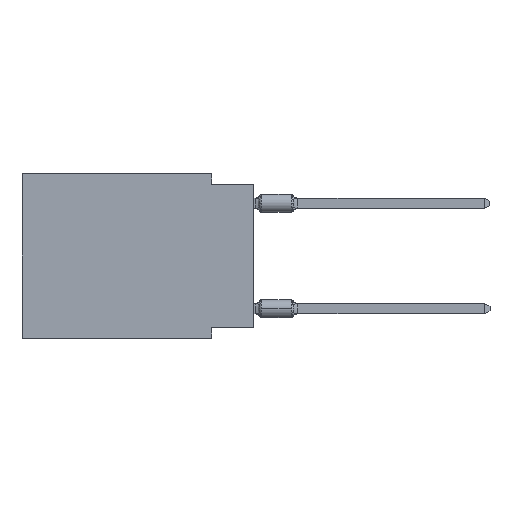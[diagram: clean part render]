
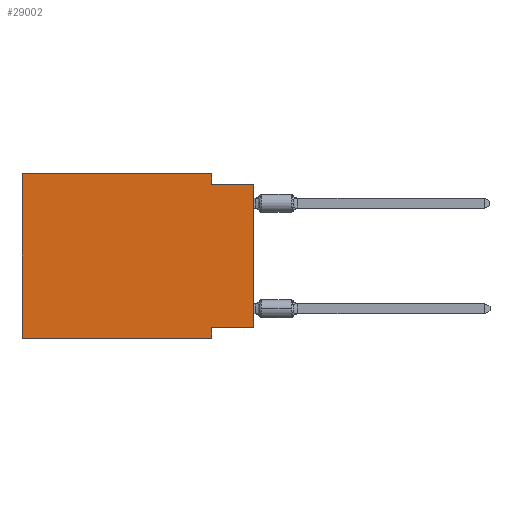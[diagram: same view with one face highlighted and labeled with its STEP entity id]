
A CAD part, left-side view. The second image highlights one B-rep face of the part: STEP entity #29002.
In plain terms, the highlighted planar face has unit normal (-1, 0, 0).
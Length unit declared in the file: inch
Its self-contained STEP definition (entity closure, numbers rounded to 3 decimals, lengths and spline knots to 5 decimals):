
#120 = CARTESIAN_POINT ( 'NONE',  ( 0., 0.1, -0.365 ) ) ;
#843 = DIRECTION ( 'NONE',  ( 0., -1., 0. ) ) ;
#1468 = CARTESIAN_POINT ( 'NONE',  ( 0., 0., -0.365 ) ) ;
#3366 = VERTEX_POINT ( 'NONE', #50216 ) ;
#4044 = LINE ( 'NONE', #29016, #26441 ) ;
#4086 = CARTESIAN_POINT ( 'NONE',  ( 0., 0., 0. ) ) ;
#5196 = CARTESIAN_POINT ( 'NONE',  ( 0., 0.55, 0. ) ) ;
#5361 = LINE ( 'NONE', #50128, #23396 ) ;
#6014 = ORIENTED_EDGE ( 'NONE', *, *, #18620, .T. ) ;
#8143 = CARTESIAN_POINT ( 'NONE',  ( 0., 0.55, 0. ) ) ;
#9577 = LINE ( 'NONE', #39129, #50438 ) ;
#12349 = ORIENTED_EDGE ( 'NONE', *, *, #35644, .F. ) ;
#12462 = VERTEX_POINT ( 'NONE', #38360 ) ;
#12705 = CARTESIAN_POINT ( 'NONE',  ( 0., 0., -0.365 ) ) ;
#13764 = DIRECTION ( 'NONE',  ( 0., 0., 1. ) ) ;
#14837 = PLANE ( 'NONE',  #52982 ) ;
#15242 = VERTEX_POINT ( 'NONE', #12705 ) ;
#15736 = LINE ( 'NONE', #8143, #47557 ) ;
#16012 = CARTESIAN_POINT ( 'NONE',  ( 0., 0.1, 0. ) ) ;
#16561 = LINE ( 'NONE', #4086, #46891 ) ;
#17152 = ORIENTED_EDGE ( 'NONE', *, *, #40180, .F. ) ;
#18620 = EDGE_CURVE ( 'NONE', #45298, #3366, #18981, .T. ) ;
#18694 = ORIENTED_EDGE ( 'NONE', *, *, #26738, .F. ) ;
#18981 = LINE ( 'NONE', #48284, #37695 ) ;
#19491 = VERTEX_POINT ( 'NONE', #22157 ) ;
#22157 = CARTESIAN_POINT ( 'NONE',  ( 0., 0.55, 0. ) ) ;
#22170 = DIRECTION ( 'NONE',  ( 0., 0., -1. ) ) ;
#22563 = ORIENTED_EDGE ( 'NONE', *, *, #23444, .F. ) ;
#23396 = VECTOR ( 'NONE', #22170, 39.37008 ) ;
#23444 = EDGE_CURVE ( 'NONE', #45298, #19491, #15736, .T. ) ;
#26441 = VECTOR ( 'NONE', #32824, 39.37008 ) ;
#26738 = EDGE_CURVE ( 'NONE', #15242, #34826, #50054, .T. ) ;
#29002 = ADVANCED_FACE ( 'NONE', ( #52019 ), #14837, .F. ) ;
#29016 = CARTESIAN_POINT ( 'NONE',  ( 0., 0.1, -0.39 ) ) ;
#30020 = ORIENTED_EDGE ( 'NONE', *, *, #44302, .T. ) ;
#30436 = ORIENTED_EDGE ( 'NONE', *, *, #43091, .F. ) ;
#30946 = DIRECTION ( 'NONE',  ( 0., -1., 0. ) ) ;
#30983 = DIRECTION ( 'NONE',  ( 0., -1., 0. ) ) ;
#30997 = VECTOR ( 'NONE', #843, 39.37008 ) ;
#31406 = DIRECTION ( 'NONE',  ( 0., 0., -1. ) ) ;
#32248 = CARTESIAN_POINT ( 'NONE',  ( 0., 0.55, -0.39 ) ) ;
#32824 = DIRECTION ( 'NONE',  ( 0., 0., -1. ) ) ;
#34826 = VERTEX_POINT ( 'NONE', #120 ) ;
#35644 = EDGE_CURVE ( 'NONE', #34826, #3366, #4044, .T. ) ;
#37206 = DIRECTION ( 'NONE',  ( 0., 0., 1. ) ) ;
#37695 = VECTOR ( 'NONE', #30946, 39.37008 ) ;
#38154 = VECTOR ( 'NONE', #50598, 39.37008 ) ;
#38360 = CARTESIAN_POINT ( 'NONE',  ( 0., 0.1, -0.025 ) ) ;
#39129 = CARTESIAN_POINT ( 'NONE',  ( 0., 0.55, 0. ) ) ;
#40180 = EDGE_CURVE ( 'NONE', #12462, #43889, #45892, .T. ) ;
#41322 = CARTESIAN_POINT ( 'NONE',  ( 0., 0., -0.025 ) ) ;
#43091 = EDGE_CURVE ( 'NONE', #46178, #12462, #5361, .T. ) ;
#43889 = VERTEX_POINT ( 'NONE', #41322 ) ;
#44302 = EDGE_CURVE ( 'NONE', #15242, #43889, #16561, .T. ) ;
#45298 = VERTEX_POINT ( 'NONE', #32248 ) ;
#45819 = EDGE_CURVE ( 'NONE', #19491, #46178, #9577, .T. ) ;
#45892 = LINE ( 'NONE', #46165, #30997 ) ;
#46161 = DIRECTION ( 'NONE',  ( 1., 0., 0. ) ) ;
#46165 = CARTESIAN_POINT ( 'NONE',  ( 0., 0., -0.025 ) ) ;
#46178 = VERTEX_POINT ( 'NONE', #16012 ) ;
#46891 = VECTOR ( 'NONE', #13764, 39.37008 ) ;
#47557 = VECTOR ( 'NONE', #37206, 39.37008 ) ;
#48284 = CARTESIAN_POINT ( 'NONE',  ( 0., 0.55, -0.39 ) ) ;
#50054 = LINE ( 'NONE', #1468, #38154 ) ;
#50128 = CARTESIAN_POINT ( 'NONE',  ( 0., 0.1, 0. ) ) ;
#50216 = CARTESIAN_POINT ( 'NONE',  ( 0., 0.1, -0.39 ) ) ;
#50438 = VECTOR ( 'NONE', #30983, 39.37008 ) ;
#50598 = DIRECTION ( 'NONE',  ( 0., 1., 0. ) ) ;
#50783 = EDGE_LOOP ( 'NONE', ( #30020, #17152, #30436, #52696, #22563, #6014, #12349, #18694 ) ) ;
#52019 = FACE_OUTER_BOUND ( 'NONE', #50783, .T. ) ;
#52696 = ORIENTED_EDGE ( 'NONE', *, *, #45819, .F. ) ;
#52982 = AXIS2_PLACEMENT_3D ( 'NONE', #5196, #46161, #31406 ) ;
